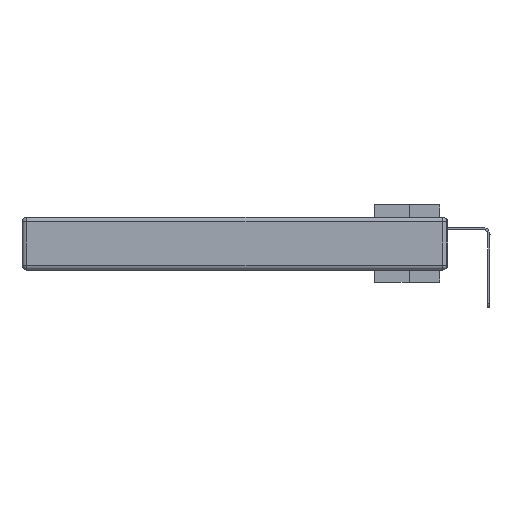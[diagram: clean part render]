
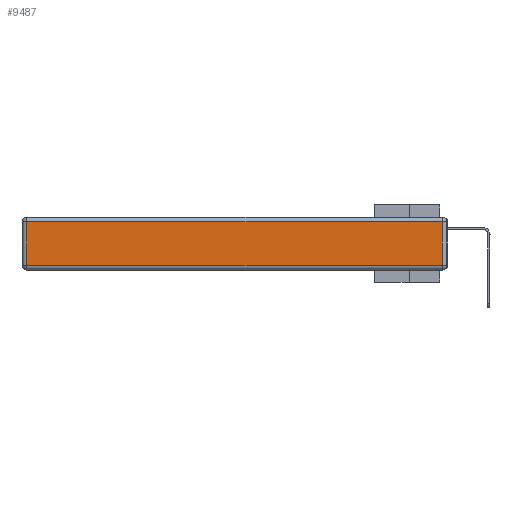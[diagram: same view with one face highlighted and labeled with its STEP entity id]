
A CAD part, left-side view. The second image highlights one B-rep face of the part: STEP entity #9487.
In plain terms, the highlighted planar face has unit normal (-1, 0, 0).
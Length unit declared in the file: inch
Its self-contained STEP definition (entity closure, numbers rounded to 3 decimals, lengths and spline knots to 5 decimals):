
#255 = CARTESIAN_POINT ( 'NONE',  ( 0., 0.03, -0.313 ) ) ;
#2697 = VERTEX_POINT ( 'NONE', #9081 ) ;
#4254 = CARTESIAN_POINT ( 'NONE',  ( 0., 2.72, -0.343 ) ) ;
#4664 = DIRECTION ( 'NONE',  ( 0., 0., 1. ) ) ;
#4736 = ORIENTED_EDGE ( 'NONE', *, *, #8106, .T. ) ;
#5914 = CARTESIAN_POINT ( 'NONE',  ( 0., 2.72, -0.03 ) ) ;
#6804 = ORIENTED_EDGE ( 'NONE', *, *, #32752, .T. ) ;
#7481 = DIRECTION ( 'NONE',  ( -1., 0., 0. ) ) ;
#7762 = CARTESIAN_POINT ( 'NONE',  ( 0., 2.75, -0.03 ) ) ;
#7875 = CARTESIAN_POINT ( 'NONE',  ( 0., 0., -0.343 ) ) ;
#7921 = VECTOR ( 'NONE', #14910, 39.37008 ) ;
#8106 = EDGE_CURVE ( 'NONE', #37828, #2697, #17586, .T. ) ;
#8953 = EDGE_LOOP ( 'NONE', ( #20966, #36897, #6804, #4736 ) ) ;
#9081 = CARTESIAN_POINT ( 'NONE',  ( 0., 2.72, -0.313 ) ) ;
#9487 = ADVANCED_FACE ( 'NONE', ( #30347 ), #13511, .T. ) ;
#11521 = VERTEX_POINT ( 'NONE', #255 ) ;
#13511 = PLANE ( 'NONE',  #26619 ) ;
#13884 = LINE ( 'NONE', #35767, #7921 ) ;
#14910 = DIRECTION ( 'NONE',  ( 0., 0., 1. ) ) ;
#16467 = LINE ( 'NONE', #7762, #38092 ) ;
#17586 = LINE ( 'NONE', #4254, #23157 ) ;
#19193 = DIRECTION ( 'NONE',  ( 0., 0., -1. ) ) ;
#20966 = ORIENTED_EDGE ( 'NONE', *, *, #34827, .T. ) ;
#21234 = EDGE_CURVE ( 'NONE', #11521, #32555, #13884, .T. ) ;
#23157 = VECTOR ( 'NONE', #19193, 39.37008 ) ;
#23708 = VECTOR ( 'NONE', #30383, 39.37008 ) ;
#24762 = CARTESIAN_POINT ( 'NONE',  ( 0., 0.03, -0.03 ) ) ;
#26619 = AXIS2_PLACEMENT_3D ( 'NONE', #7875, #7481, #4664 ) ;
#30347 = FACE_OUTER_BOUND ( 'NONE', #8953, .T. ) ;
#30383 = DIRECTION ( 'NONE',  ( 0., -1., 0. ) ) ;
#31955 = LINE ( 'NONE', #33220, #23708 ) ;
#32555 = VERTEX_POINT ( 'NONE', #24762 ) ;
#32752 = EDGE_CURVE ( 'NONE', #32555, #37828, #16467, .T. ) ;
#33220 = CARTESIAN_POINT ( 'NONE',  ( 0., 0., -0.313 ) ) ;
#34827 = EDGE_CURVE ( 'NONE', #2697, #11521, #31955, .T. ) ;
#35767 = CARTESIAN_POINT ( 'NONE',  ( 0., 0.03, -0.343 ) ) ;
#36897 = ORIENTED_EDGE ( 'NONE', *, *, #21234, .T. ) ;
#37352 = DIRECTION ( 'NONE',  ( 0., 1., 0. ) ) ;
#37828 = VERTEX_POINT ( 'NONE', #5914 ) ;
#38092 = VECTOR ( 'NONE', #37352, 39.37008 ) ;
